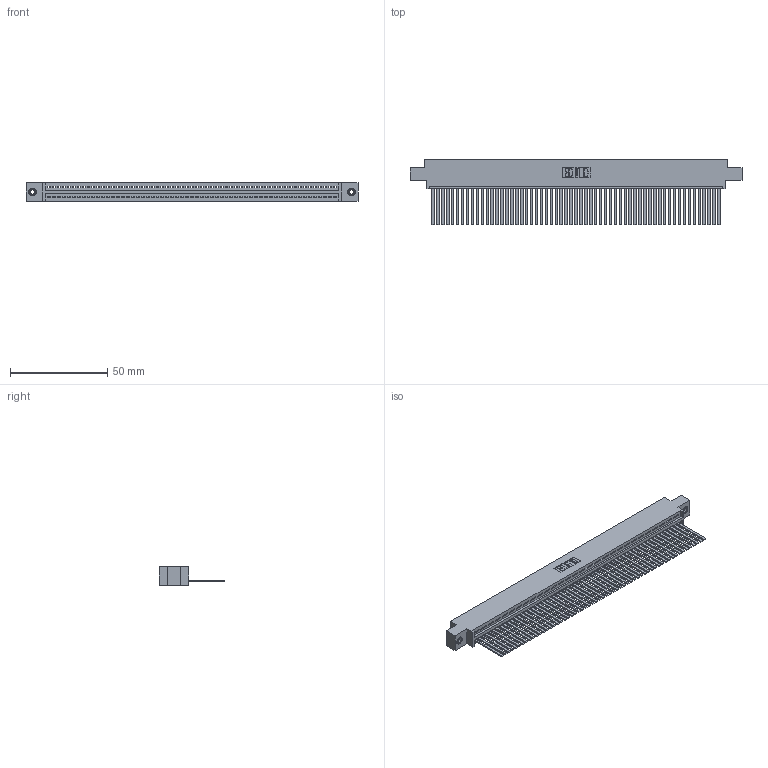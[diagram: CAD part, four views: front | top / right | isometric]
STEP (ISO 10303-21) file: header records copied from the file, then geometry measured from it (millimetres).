
FILE_DESCRIPTION (( 'STEP AP203' ), '1' );
FILE_NAME ('395-059-544-608.STEP', '2018-11-23T09:30:38', ( '' ), ( '' ), 'SwSTEP 2.0', 'SolidWorks 2016', '' );
FILE_SCHEMA (( 'CONFIG_CONTROL_DESIGN' ));
Length unit declared in the file: inch
Products named in the file (4): 345 Part_0.170 Offset - 0.156 Dia-TI; 345-292-001_345-293-144; 395-059-544-608; 345-250-001_345-250-003-102
Assembly tree (62 placements, depth 2):
  395-059-544-608
    345 Part_0.170 Offset - 0.156 Dia-TI
    345-292-001_345-293-144  x59
    345-250-001_345-250-003-102  x2
Bounding box: 171.07 x 33.96 x 9.4 mm (x, y, z)
Volume: 16951 mm3; surface area: 24954.4 mm2
Topology: 62 solids, 62 shells, 3258 faces, 9811 edges, 6454 vertices
Faces by surface type: plane 2240, cylinder 1002, cone 12, torus 4
Entity records: 43250 total; most frequent: CARTESIAN_POINT 7472, ORIENTED_EDGE 7458, DIRECTION 6525, EDGE_CURVE 3729, VECTOR 3345, LINE 3345, VERTEX_POINT 2480, AXIS2_PLACEMENT_3D 1590
